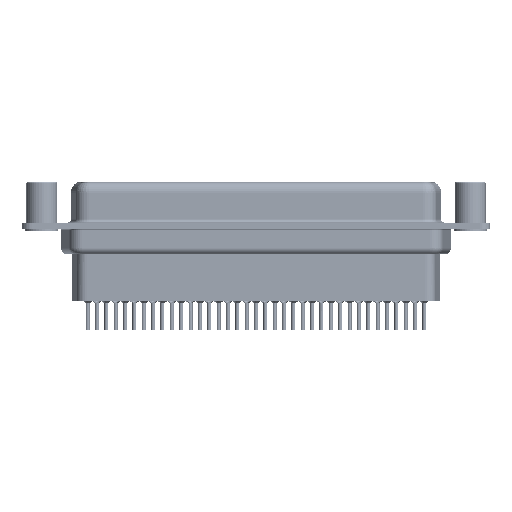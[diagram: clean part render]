
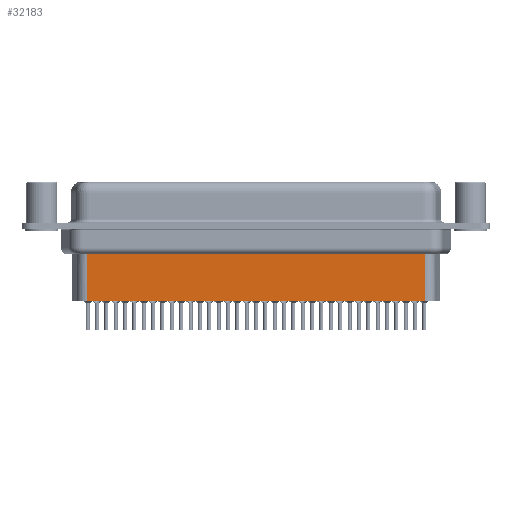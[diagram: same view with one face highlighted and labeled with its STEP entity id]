
A CAD part, front view. The second image highlights one B-rep face of the part: STEP entity #32183.
In plain terms, the highlighted planar face has unit normal (0, -1, 0).
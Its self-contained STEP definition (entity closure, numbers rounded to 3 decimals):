
#15 = EDGE_CURVE ( 'NONE', #13929, #5372, #27441, .T. ) ;
#667 = CARTESIAN_POINT ( 'NONE',  ( 56.794, -3.5, -11.15 ) ) ;
#2744 = ORIENTED_EDGE ( 'NONE', *, *, #15334, .T. ) ;
#2765 = PLANE ( 'NONE',  #30348 ) ;
#3529 = EDGE_CURVE ( 'NONE', #5372, #21236, #23765, .T. ) ;
#5372 = VERTEX_POINT ( 'NONE', #667 ) ;
#8619 = VECTOR ( 'NONE', #29505, 1000. ) ;
#9277 = ORIENTED_EDGE ( 'NONE', *, *, #12419, .T. ) ;
#10790 = ORIENTED_EDGE ( 'NONE', *, *, #3529, .F. ) ;
#11048 = DIRECTION ( 'NONE',  ( 0., 0., -1. ) ) ;
#11223 = CARTESIAN_POINT ( 'NONE',  ( 56.794, -3.5, -4.097 ) ) ;
#11301 = VECTOR ( 'NONE', #24551, 1000. ) ;
#11701 = DIRECTION ( 'NONE',  ( 0., 0., -1. ) ) ;
#12419 = EDGE_CURVE ( 'NONE', #24807, #21236, #31365, .T. ) ;
#13614 = CARTESIAN_POINT ( 'NONE',  ( 6.706, -3.5, -3.1 ) ) ;
#13929 = VERTEX_POINT ( 'NONE', #11223 ) ;
#14232 = CARTESIAN_POINT ( 'NONE',  ( 6.459, -3.5, -4.097 ) ) ;
#14952 = VECTOR ( 'NONE', #11701, 1000. ) ;
#15334 = EDGE_CURVE ( 'NONE', #13929, #24807, #17444, .T. ) ;
#16171 = DIRECTION ( 'NONE',  ( 1., 0., 0. ) ) ;
#16326 = CARTESIAN_POINT ( 'NONE',  ( 6.706, -3.5, -11.15 ) ) ;
#17125 = CARTESIAN_POINT ( 'NONE',  ( 56.794, -3.5, -3.1 ) ) ;
#17127 = VECTOR ( 'NONE', #11048, 1000. ) ;
#17444 = LINE ( 'NONE', #14232, #11301 ) ;
#18075 = ORIENTED_EDGE ( 'NONE', *, *, #15, .F. ) ;
#21075 = CARTESIAN_POINT ( 'NONE',  ( 6.706, -3.5, -11.15 ) ) ;
#21236 = VERTEX_POINT ( 'NONE', #21075 ) ;
#21587 = CARTESIAN_POINT ( 'NONE',  ( 6.706, -3.5, -4.097 ) ) ;
#22075 = EDGE_LOOP ( 'NONE', ( #18075, #2744, #9277, #10790 ) ) ;
#23765 = LINE ( 'NONE', #16326, #8619 ) ;
#23946 = FACE_OUTER_BOUND ( 'NONE', #22075, .T. ) ;
#24551 = DIRECTION ( 'NONE',  ( -1., 0., 0. ) ) ;
#24807 = VERTEX_POINT ( 'NONE', #21587 ) ;
#27441 = LINE ( 'NONE', #17125, #14952 ) ;
#28823 = CARTESIAN_POINT ( 'NONE',  ( 6.706, -3.5, -3.1 ) ) ;
#29041 = DIRECTION ( 'NONE',  ( 0., -1., 0. ) ) ;
#29505 = DIRECTION ( 'NONE',  ( -1., 0., 0. ) ) ;
#30348 = AXIS2_PLACEMENT_3D ( 'NONE', #13614, #29041, #16171 ) ;
#31365 = LINE ( 'NONE', #28823, #17127 ) ;
#32183 = ADVANCED_FACE ( 'NONE', ( #23946 ), #2765, .T. ) ;
